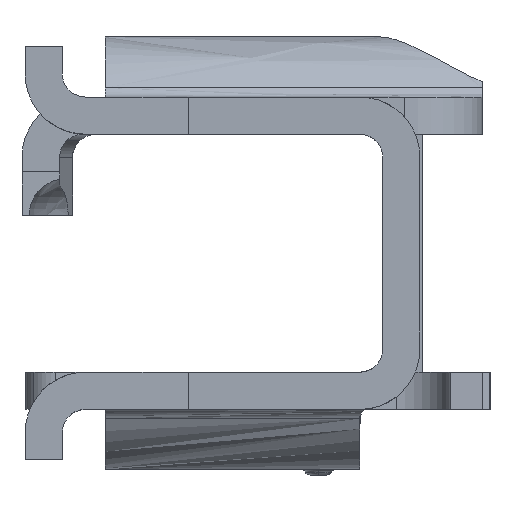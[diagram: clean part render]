
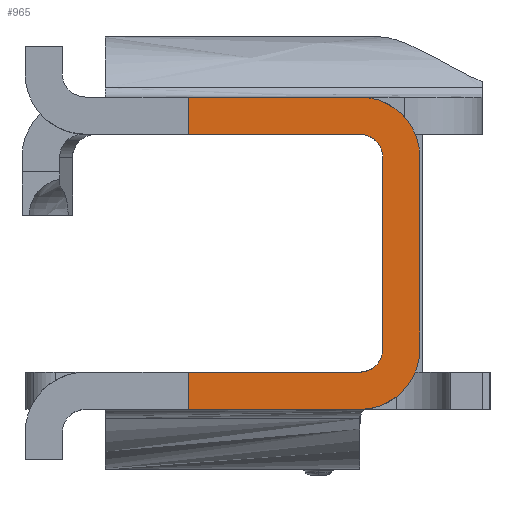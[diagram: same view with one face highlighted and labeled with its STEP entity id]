
A CAD part, left-side view. The second image highlights one B-rep face of the part: STEP entity #965.
In plain terms, the highlighted planar face has unit normal (-1, 0, 0).
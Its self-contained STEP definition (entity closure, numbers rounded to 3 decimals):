
#3 = CARTESIAN_POINT ( 'NONE',  ( -11.5, 5.313, 0. ) ) ;
#57 = CARTESIAN_POINT ( 'NONE',  ( -11.5, -5.934, -7.287 ) ) ;
#65 = ORIENTED_EDGE ( 'NONE', *, *, #5694, .F. ) ;
#147 = CARTESIAN_POINT ( 'NONE',  ( -11.5, -3.689, 5.042 ) ) ;
#159 = VECTOR ( 'NONE', #7808, 1000. ) ;
#237 = VERTEX_POINT ( 'NONE', #7306 ) ;
#240 = LINE ( 'NONE', #6178, #5205 ) ;
#256 = ORIENTED_EDGE ( 'NONE', *, *, #290, .F. ) ;
#282 = CARTESIAN_POINT ( 'NONE',  ( -11.5, -4.909, 5.042 ) ) ;
#290 = EDGE_CURVE ( 'NONE', #6441, #237, #343, .T. ) ;
#339 = CIRCLE ( 'NONE', #5178, 1.219 ) ;
#343 = CIRCLE ( 'NONE', #6079, 1.219 ) ;
#363 = CARTESIAN_POINT ( 'NONE',  ( -11.5, -4.551, -5.904 ) ) ;
#440 = CARTESIAN_POINT ( 'NONE',  ( -11.5, -3.689, -6.261 ) ) ;
#624 = PLANE ( 'NONE',  #5156 ) ;
#795 = DIRECTION ( 'NONE',  ( 0., -0.707, 0.707 ) ) ;
#857 = ORIENTED_EDGE ( 'NONE', *, *, #6734, .T. ) ;
#875 = CARTESIAN_POINT ( 'NONE',  ( -11.5, -5.934, 7.287 ) ) ;
#904 = CIRCLE ( 'NONE', #6699, 1.219 ) ;
#919 = DIRECTION ( 'NONE',  ( 1., 0., 0. ) ) ;
#934 = DIRECTION ( 'NONE',  ( -1., 0., 0. ) ) ;
#938 = LINE ( 'NONE', #7054, #2457 ) ;
#946 = ORIENTED_EDGE ( 'NONE', *, *, #6417, .F. ) ;
#965 = ADVANCED_FACE ( 'NONE', ( #7855 ), #624, .T. ) ;
#1067 = CARTESIAN_POINT ( 'NONE',  ( -11.5, -6.864, 5.042 ) ) ;
#1075 = EDGE_CURVE ( 'NONE', #1800, #7977, #3385, .T. ) ;
#1333 = EDGE_CURVE ( 'NONE', #3901, #3386, #240, .T. ) ;
#1341 = CARTESIAN_POINT ( 'NONE',  ( -11.5, -3.689, 8.217 ) ) ;
#1403 = DIRECTION ( 'NONE',  ( -1., 0., 0. ) ) ;
#1405 = VERTEX_POINT ( 'NONE', #1067 ) ;
#1484 = LINE ( 'NONE', #3473, #6457 ) ;
#1485 = CARTESIAN_POINT ( 'NONE',  ( -11.5, 2.928, 8.217 ) ) ;
#1495 = EDGE_CURVE ( 'NONE', #4358, #237, #938, .T. ) ;
#1537 = CIRCLE ( 'NONE', #7744, 1.219 ) ;
#1574 = CARTESIAN_POINT ( 'NONE',  ( -11.5, 0.202, -6.261 ) ) ;
#1621 = DIRECTION ( 'NONE',  ( 1., 0., 0. ) ) ;
#1657 = VECTOR ( 'NONE', #4711, 1000. ) ;
#1659 = DIRECTION ( 'NONE',  ( 0., 0., -1. ) ) ;
#1800 = VERTEX_POINT ( 'NONE', #1341 ) ;
#1953 = DIRECTION ( 'NONE',  ( -1., 0., 0. ) ) ;
#2033 = VERTEX_POINT ( 'NONE', #3866 ) ;
#2128 = ORIENTED_EDGE ( 'NONE', *, *, #1333, .T. ) ;
#2137 = CARTESIAN_POINT ( 'NONE',  ( -11.5, -6.864, 0. ) ) ;
#2142 = VECTOR ( 'NONE', #2801, 1000. ) ;
#2212 = DIRECTION ( 'NONE',  ( 0., 1., 0. ) ) ;
#2341 = CARTESIAN_POINT ( 'NONE',  ( -11.5, -3.689, 5.042 ) ) ;
#2457 = VECTOR ( 'NONE', #3152, 1000. ) ;
#2505 = CARTESIAN_POINT ( 'NONE',  ( -11.5, -3.689, 6.261 ) ) ;
#2541 = CARTESIAN_POINT ( 'NONE',  ( -11.5, 5.313, 0. ) ) ;
#2656 = DIRECTION ( 'NONE',  ( 1., 0., 0. ) ) ;
#2690 = EDGE_LOOP ( 'NONE', ( #4255, #4154, #5757, #7531, #3767, #7494, #857, #3880, #65, #4312, #256, #946, #5336, #2128, #5469, #3622 ) ) ;
#2701 = CIRCLE ( 'NONE', #5289, 3.175 ) ;
#2738 = EDGE_CURVE ( 'NONE', #8131, #3901, #8316, .T. ) ;
#2760 = EDGE_CURVE ( 'NONE', #8360, #7064, #5077, .T. ) ;
#2801 = DIRECTION ( 'NONE',  ( 0., 0., 1. ) ) ;
#2931 = CARTESIAN_POINT ( 'NONE',  ( -11.5, -3.689, -5.042 ) ) ;
#2999 = DIRECTION ( 'NONE',  ( 0., -0.707, 0.707 ) ) ;
#3041 = EDGE_CURVE ( 'NONE', #3815, #8264, #904, .T. ) ;
#3142 = VERTEX_POINT ( 'NONE', #875 ) ;
#3152 = DIRECTION ( 'NONE',  ( 0., 0., -1. ) ) ;
#3192 = CARTESIAN_POINT ( 'NONE',  ( -11.5, -3.689, -8.217 ) ) ;
#3385 = LINE ( 'NONE', #1485, #1657 ) ;
#3386 = VERTEX_POINT ( 'NONE', #5659 ) ;
#3473 = CARTESIAN_POINT ( 'NONE',  ( -11.5, 2.928, -8.217 ) ) ;
#3584 = DIRECTION ( 'NONE',  ( 0., -0.707, -0.707 ) ) ;
#3622 = ORIENTED_EDGE ( 'NONE', *, *, #4260, .F. ) ;
#3761 = AXIS2_PLACEMENT_3D ( 'NONE', #4824, #919, #5456 ) ;
#3767 = ORIENTED_EDGE ( 'NONE', *, *, #1075, .T. ) ;
#3815 = VERTEX_POINT ( 'NONE', #4436 ) ;
#3822 = AXIS2_PLACEMENT_3D ( 'NONE', #2341, #6894, #2999 ) ;
#3866 = CARTESIAN_POINT ( 'NONE',  ( -11.5, 5.313, 6.261 ) ) ;
#3880 = ORIENTED_EDGE ( 'NONE', *, *, #3041, .F. ) ;
#3901 = VERTEX_POINT ( 'NONE', #5197 ) ;
#3927 = CARTESIAN_POINT ( 'NONE',  ( -11.5, 9.606, 6.261 ) ) ;
#4069 = LINE ( 'NONE', #2137, #2142 ) ;
#4154 = ORIENTED_EDGE ( 'NONE', *, *, #6305, .T. ) ;
#4255 = ORIENTED_EDGE ( 'NONE', *, *, #2760, .F. ) ;
#4260 = EDGE_CURVE ( 'NONE', #7064, #6678, #2701, .T. ) ;
#4285 = VECTOR ( 'NONE', #4469, 1000. ) ;
#4312 = ORIENTED_EDGE ( 'NONE', *, *, #1495, .T. ) ;
#4358 = VERTEX_POINT ( 'NONE', #282 ) ;
#4436 = CARTESIAN_POINT ( 'NONE',  ( -11.5, -4.551, 5.904 ) ) ;
#4469 = DIRECTION ( 'NONE',  ( 0., 0., -1. ) ) ;
#4501 = LINE ( 'NONE', #2541, #4285 ) ;
#4511 = EDGE_CURVE ( 'NONE', #3142, #1405, #4524, .T. ) ;
#4524 = CIRCLE ( 'NONE', #3822, 3.175 ) ;
#4676 = DIRECTION ( 'NONE',  ( -1., 0., 0. ) ) ;
#4699 = CIRCLE ( 'NONE', #3761, 3.175 ) ;
#4711 = DIRECTION ( 'NONE',  ( 0., 1., 0. ) ) ;
#4824 = CARTESIAN_POINT ( 'NONE',  ( -11.5, -3.689, 5.042 ) ) ;
#4830 = CARTESIAN_POINT ( 'NONE',  ( -11.5, -3.689, -5.042 ) ) ;
#4915 = EDGE_CURVE ( 'NONE', #3386, #6678, #1484, .T. ) ;
#5077 = CIRCLE ( 'NONE', #5758, 3.175 ) ;
#5107 = EDGE_CURVE ( 'NONE', #1800, #3142, #4699, .T. ) ;
#5156 = AXIS2_PLACEMENT_3D ( 'NONE', #3, #1953, #6503 ) ;
#5178 = AXIS2_PLACEMENT_3D ( 'NONE', #5276, #1403, #5935 ) ;
#5197 = CARTESIAN_POINT ( 'NONE',  ( -11.5, 5.313, -6.261 ) ) ;
#5205 = VECTOR ( 'NONE', #1659, 1000. ) ;
#5276 = CARTESIAN_POINT ( 'NONE',  ( -11.5, -3.689, 5.042 ) ) ;
#5289 = AXIS2_PLACEMENT_3D ( 'NONE', #6568, #2656, #7205 ) ;
#5336 = ORIENTED_EDGE ( 'NONE', *, *, #2738, .T. ) ;
#5456 = DIRECTION ( 'NONE',  ( 0., -0.707, 0.707 ) ) ;
#5464 = DIRECTION ( 'NONE',  ( 0., -0.707, -0.707 ) ) ;
#5469 = ORIENTED_EDGE ( 'NONE', *, *, #4915, .T. ) ;
#5499 = CARTESIAN_POINT ( 'NONE',  ( -11.5, -3.689, -5.042 ) ) ;
#5659 = CARTESIAN_POINT ( 'NONE',  ( -11.5, 5.313, -8.217 ) ) ;
#5694 = EDGE_CURVE ( 'NONE', #4358, #3815, #339, .T. ) ;
#5757 = ORIENTED_EDGE ( 'NONE', *, *, #4511, .F. ) ;
#5758 = AXIS2_PLACEMENT_3D ( 'NONE', #5499, #1621, #6172 ) ;
#5935 = DIRECTION ( 'NONE',  ( 0., -0.707, 0.707 ) ) ;
#6070 = CARTESIAN_POINT ( 'NONE',  ( -11.5, 5.313, 8.217 ) ) ;
#6079 = AXIS2_PLACEMENT_3D ( 'NONE', #4830, #934, #5464 ) ;
#6172 = DIRECTION ( 'NONE',  ( 0., -0.707, -0.707 ) ) ;
#6178 = CARTESIAN_POINT ( 'NONE',  ( -11.5, 5.313, 0. ) ) ;
#6305 = EDGE_CURVE ( 'NONE', #8360, #1405, #4069, .T. ) ;
#6417 = EDGE_CURVE ( 'NONE', #8131, #6441, #1537, .T. ) ;
#6441 = VERTEX_POINT ( 'NONE', #363 ) ;
#6457 = VECTOR ( 'NONE', #6717, 1000. ) ;
#6503 = DIRECTION ( 'NONE',  ( 0., -1., 0. ) ) ;
#6568 = CARTESIAN_POINT ( 'NONE',  ( -11.5, -3.689, -5.042 ) ) ;
#6611 = VECTOR ( 'NONE', #2212, 1000. ) ;
#6662 = LINE ( 'NONE', #3927, #159 ) ;
#6678 = VERTEX_POINT ( 'NONE', #3192 ) ;
#6699 = AXIS2_PLACEMENT_3D ( 'NONE', #147, #4676, #795 ) ;
#6717 = DIRECTION ( 'NONE',  ( 0., -1., 0. ) ) ;
#6734 = EDGE_CURVE ( 'NONE', #2033, #8264, #6662, .T. ) ;
#6894 = DIRECTION ( 'NONE',  ( 1., 0., 0. ) ) ;
#7054 = CARTESIAN_POINT ( 'NONE',  ( -11.5, -4.909, 3.131 ) ) ;
#7064 = VERTEX_POINT ( 'NONE', #57 ) ;
#7205 = DIRECTION ( 'NONE',  ( 0., -0.707, -0.707 ) ) ;
#7291 = CARTESIAN_POINT ( 'NONE',  ( -11.5, -6.864, -5.042 ) ) ;
#7306 = CARTESIAN_POINT ( 'NONE',  ( -11.5, -4.909, -5.042 ) ) ;
#7480 = DIRECTION ( 'NONE',  ( -1., 0., 0. ) ) ;
#7494 = ORIENTED_EDGE ( 'NONE', *, *, #7700, .T. ) ;
#7531 = ORIENTED_EDGE ( 'NONE', *, *, #5107, .F. ) ;
#7700 = EDGE_CURVE ( 'NONE', #7977, #2033, #4501, .T. ) ;
#7744 = AXIS2_PLACEMENT_3D ( 'NONE', #2931, #7480, #3584 ) ;
#7808 = DIRECTION ( 'NONE',  ( 0., -1., 0. ) ) ;
#7855 = FACE_OUTER_BOUND ( 'NONE', #2690, .T. ) ;
#7977 = VERTEX_POINT ( 'NONE', #6070 ) ;
#8131 = VERTEX_POINT ( 'NONE', #440 ) ;
#8264 = VERTEX_POINT ( 'NONE', #2505 ) ;
#8316 = LINE ( 'NONE', #1574, #6611 ) ;
#8360 = VERTEX_POINT ( 'NONE', #7291 ) ;
